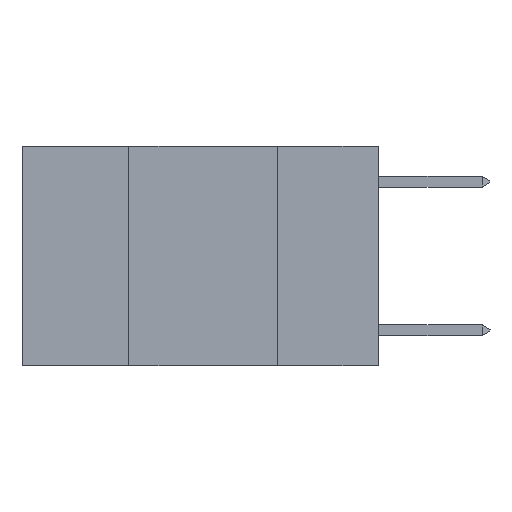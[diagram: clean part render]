
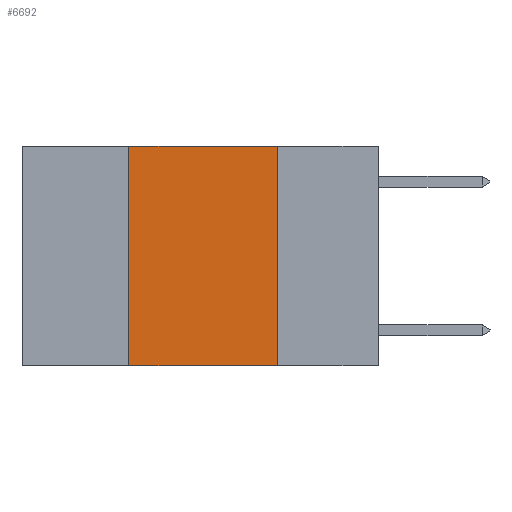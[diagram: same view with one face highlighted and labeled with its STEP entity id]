
A CAD part, left-side view. The second image highlights one B-rep face of the part: STEP entity #6692.
In plain terms, the highlighted planar face has unit normal (-1, 0, 0).
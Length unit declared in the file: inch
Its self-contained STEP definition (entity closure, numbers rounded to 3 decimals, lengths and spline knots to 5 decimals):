
#1481 = VERTEX_POINT ( 'NONE', #8789 ) ;
#2659 = VECTOR ( 'NONE', #5425, 39.37008 ) ;
#2738 = LINE ( 'NONE', #3523, #2659 ) ;
#3523 = CARTESIAN_POINT ( 'NONE',  ( 0., 0.6, -0.37 ) ) ;
#3926 = CARTESIAN_POINT ( 'NONE',  ( 0., 0.42, 0. ) ) ;
#4663 = EDGE_CURVE ( 'NONE', #15733, #17400, #2738, .T. ) ;
#5027 = DIRECTION ( 'NONE',  ( 1., 0., 0. ) ) ;
#5425 = DIRECTION ( 'NONE',  ( 0., -1., 0. ) ) ;
#5927 = EDGE_CURVE ( 'NONE', #15733, #21803, #6899, .T. ) ;
#6060 = CARTESIAN_POINT ( 'NONE',  ( 0., 0.17, 0. ) ) ;
#6692 = ADVANCED_FACE ( 'NONE', ( #20469 ), #15766, .F. ) ;
#6775 = VECTOR ( 'NONE', #12474, 39.37008 ) ;
#6899 = LINE ( 'NONE', #12066, #7160 ) ;
#6912 = LINE ( 'NONE', #7020, #6775 ) ;
#7020 = CARTESIAN_POINT ( 'NONE',  ( 0., 0.6, 0. ) ) ;
#7140 = EDGE_CURVE ( 'NONE', #1481, #17400, #17880, .T. ) ;
#7160 = VECTOR ( 'NONE', #15606, 39.37008 ) ;
#7712 = EDGE_LOOP ( 'NONE', ( #16980, #17230, #17714, #17793 ) ) ;
#7972 = DIRECTION ( 'NONE',  ( 0., 0., -1. ) ) ;
#8789 = CARTESIAN_POINT ( 'NONE',  ( 0., 0.17, 0. ) ) ;
#8856 = EDGE_CURVE ( 'NONE', #21803, #1481, #6912, .T. ) ;
#10481 = CARTESIAN_POINT ( 'NONE',  ( 0., 0.6, 0. ) ) ;
#12066 = CARTESIAN_POINT ( 'NONE',  ( 0., 0.42, 0. ) ) ;
#12474 = DIRECTION ( 'NONE',  ( 0., -1., 0. ) ) ;
#15606 = DIRECTION ( 'NONE',  ( 0., 0., 1. ) ) ;
#15733 = VERTEX_POINT ( 'NONE', #16407 ) ;
#15766 = PLANE ( 'NONE',  #20992 ) ;
#16407 = CARTESIAN_POINT ( 'NONE',  ( 0., 0.42, -0.37 ) ) ;
#16980 = ORIENTED_EDGE ( 'NONE', *, *, #7140, .F. ) ;
#17230 = ORIENTED_EDGE ( 'NONE', *, *, #8856, .F. ) ;
#17400 = VERTEX_POINT ( 'NONE', #18286 ) ;
#17714 = ORIENTED_EDGE ( 'NONE', *, *, #5927, .F. ) ;
#17722 = DIRECTION ( 'NONE',  ( 0., 0., -1. ) ) ;
#17793 = ORIENTED_EDGE ( 'NONE', *, *, #4663, .T. ) ;
#17874 = VECTOR ( 'NONE', #7972, 39.37008 ) ;
#17880 = LINE ( 'NONE', #6060, #17874 ) ;
#18286 = CARTESIAN_POINT ( 'NONE',  ( 0., 0.17, -0.37 ) ) ;
#20469 = FACE_OUTER_BOUND ( 'NONE', #7712, .T. ) ;
#20992 = AXIS2_PLACEMENT_3D ( 'NONE', #10481, #5027, #17722 ) ;
#21803 = VERTEX_POINT ( 'NONE', #3926 ) ;
